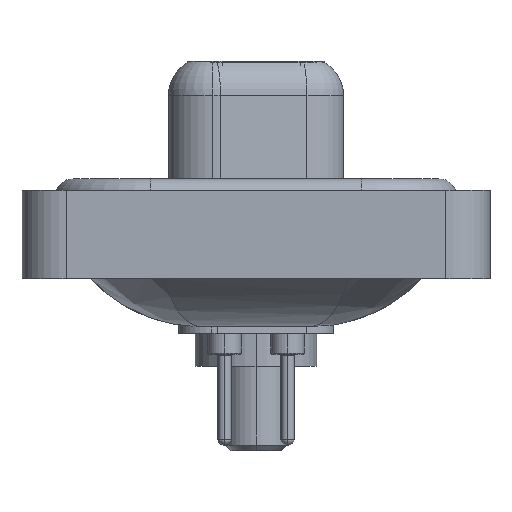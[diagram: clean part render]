
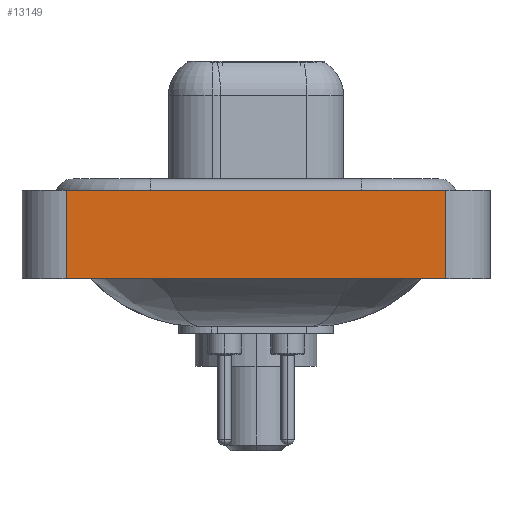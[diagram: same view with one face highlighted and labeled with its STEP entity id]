
A CAD part, left-side view. The second image highlights one B-rep face of the part: STEP entity #13149.
In plain terms, the highlighted planar face has unit normal (-1, 0, 0).
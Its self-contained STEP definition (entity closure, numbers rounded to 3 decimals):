
#214 = LINE ( 'NONE', #6263, #16479 ) ;
#997 = CARTESIAN_POINT ( 'NONE',  ( -7.25, -8.55, -3.6 ) ) ;
#1085 = DIRECTION ( 'NONE',  ( -1., 0., 0. ) ) ;
#1129 = VERTEX_POINT ( 'NONE', #2575 ) ;
#1495 = DIRECTION ( 'NONE',  ( 0., -1., 0. ) ) ;
#2575 = CARTESIAN_POINT ( 'NONE',  ( -7.25, 8.55, -3.6 ) ) ;
#2633 = VERTEX_POINT ( 'NONE', #13198 ) ;
#3854 = ORIENTED_EDGE ( 'NONE', *, *, #12201, .F. ) ;
#4059 = PLANE ( 'NONE',  #18578 ) ;
#4656 = LINE ( 'NONE', #17020, #17326 ) ;
#4779 = DIRECTION ( 'NONE',  ( 0., 0., 1. ) ) ;
#4961 = EDGE_LOOP ( 'NONE', ( #18844, #17638, #3854, #13035 ) ) ;
#5272 = FACE_OUTER_BOUND ( 'NONE', #4961, .T. ) ;
#5307 = VECTOR ( 'NONE', #1495, 1000. ) ;
#5978 = LINE ( 'NONE', #14987, #5307 ) ;
#6263 = CARTESIAN_POINT ( 'NONE',  ( -7.25, 8.55, -3.6 ) ) ;
#7680 = DIRECTION ( 'NONE',  ( 0., -1., 0. ) ) ;
#7689 = VERTEX_POINT ( 'NONE', #12128 ) ;
#10044 = VERTEX_POINT ( 'NONE', #12444 ) ;
#12128 = CARTESIAN_POINT ( 'NONE',  ( -7.25, -8.55, -3.6 ) ) ;
#12201 = EDGE_CURVE ( 'NONE', #1129, #2633, #214, .T. ) ;
#12444 = CARTESIAN_POINT ( 'NONE',  ( -7.25, -8.55, 0.4 ) ) ;
#13035 = ORIENTED_EDGE ( 'NONE', *, *, #19039, .T. ) ;
#13149 = ADVANCED_FACE ( 'NONE', ( #5272 ), #4059, .T. ) ;
#13198 = CARTESIAN_POINT ( 'NONE',  ( -7.25, 8.55, 0.4 ) ) ;
#13786 = CARTESIAN_POINT ( 'NONE',  ( -7.25, -8.55, -3.6 ) ) ;
#14139 = EDGE_CURVE ( 'NONE', #2633, #10044, #5978, .T. ) ;
#14617 = VECTOR ( 'NONE', #4779, 1000. ) ;
#14987 = CARTESIAN_POINT ( 'NONE',  ( -7.25, -8.55, 0.4 ) ) ;
#16479 = VECTOR ( 'NONE', #18530, 1000. ) ;
#17020 = CARTESIAN_POINT ( 'NONE',  ( -7.25, -8.55, -3.6 ) ) ;
#17325 = DIRECTION ( 'NONE',  ( 0., 0., 1. ) ) ;
#17326 = VECTOR ( 'NONE', #7680, 1000. ) ;
#17638 = ORIENTED_EDGE ( 'NONE', *, *, #14139, .F. ) ;
#17840 = EDGE_CURVE ( 'NONE', #7689, #10044, #18321, .T. ) ;
#18321 = LINE ( 'NONE', #13786, #14617 ) ;
#18530 = DIRECTION ( 'NONE',  ( 0., 0., 1. ) ) ;
#18578 = AXIS2_PLACEMENT_3D ( 'NONE', #997, #1085, #17325 ) ;
#18844 = ORIENTED_EDGE ( 'NONE', *, *, #17840, .T. ) ;
#19039 = EDGE_CURVE ( 'NONE', #1129, #7689, #4656, .T. ) ;
